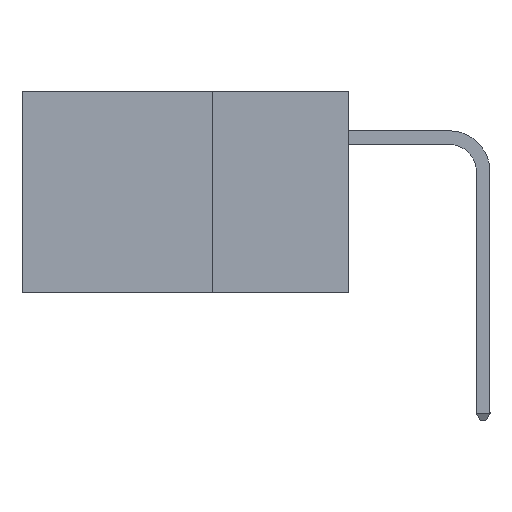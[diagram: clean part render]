
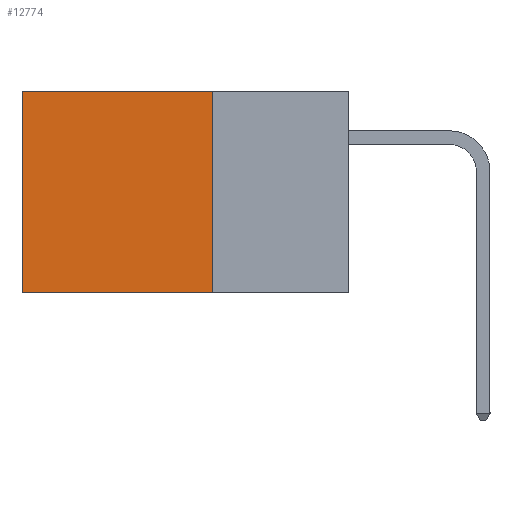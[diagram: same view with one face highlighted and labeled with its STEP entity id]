
A CAD part, left-side view. The second image highlights one B-rep face of the part: STEP entity #12774.
In plain terms, the highlighted planar face has unit normal (-1, 0, 0).
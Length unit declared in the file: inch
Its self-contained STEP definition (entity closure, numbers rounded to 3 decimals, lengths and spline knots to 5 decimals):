
#1997 = ORIENTED_EDGE ( 'NONE', *, *, #27370, .F. ) ;
#2489 = LINE ( 'NONE', #37557, #10954 ) ;
#5435 = CARTESIAN_POINT ( 'NONE',  ( 0.2875, 0.6, 0. ) ) ;
#5559 = VECTOR ( 'NONE', #21920, 39.37008 ) ;
#6791 = LINE ( 'NONE', #9286, #37528 ) ;
#7188 = AXIS2_PLACEMENT_3D ( 'NONE', #17265, #32128, #8507 ) ;
#7825 = EDGE_CURVE ( 'NONE', #21412, #36766, #33072, .T. ) ;
#8507 = DIRECTION ( 'NONE',  ( 0., 0., -1. ) ) ;
#9286 = CARTESIAN_POINT ( 'NONE',  ( 0.2875, 0.25, 0. ) ) ;
#10276 = CARTESIAN_POINT ( 'NONE',  ( 0.2875, 0.6, 0. ) ) ;
#10954 = VECTOR ( 'NONE', #14282, 39.37008 ) ;
#12774 = ADVANCED_FACE ( 'NONE', ( #19573 ), #25663, .F. ) ;
#14282 = DIRECTION ( 'NONE',  ( 0., 1., 0. ) ) ;
#15362 = EDGE_CURVE ( 'NONE', #36766, #19641, #24756, .T. ) ;
#17265 = CARTESIAN_POINT ( 'NONE',  ( 0.2875, 0.25, 0. ) ) ;
#18591 = DIRECTION ( 'NONE',  ( 0., 0., -1. ) ) ;
#19573 = FACE_OUTER_BOUND ( 'NONE', #32925, .T. ) ;
#19641 = VERTEX_POINT ( 'NONE', #34172 ) ;
#21412 = VERTEX_POINT ( 'NONE', #26914 ) ;
#21839 = CARTESIAN_POINT ( 'NONE',  ( 0.2875, 0.25, 0. ) ) ;
#21920 = DIRECTION ( 'NONE',  ( 0., 0., -1. ) ) ;
#23486 = EDGE_CURVE ( 'NONE', #21412, #24612, #6791, .T. ) ;
#24084 = ORIENTED_EDGE ( 'NONE', *, *, #23486, .F. ) ;
#24612 = VERTEX_POINT ( 'NONE', #30520 ) ;
#24756 = LINE ( 'NONE', #10276, #5559 ) ;
#25663 = PLANE ( 'NONE',  #7188 ) ;
#26505 = ORIENTED_EDGE ( 'NONE', *, *, #7825, .T. ) ;
#26914 = CARTESIAN_POINT ( 'NONE',  ( 0.2875, 0.25, 0. ) ) ;
#27370 = EDGE_CURVE ( 'NONE', #24612, #19641, #2489, .T. ) ;
#30520 = CARTESIAN_POINT ( 'NONE',  ( 0.2875, 0.25, -0.37 ) ) ;
#32128 = DIRECTION ( 'NONE',  ( 1., 0., 0. ) ) ;
#32925 = EDGE_LOOP ( 'NONE', ( #34605, #1997, #24084, #26505 ) ) ;
#33072 = LINE ( 'NONE', #21839, #36279 ) ;
#33633 = DIRECTION ( 'NONE',  ( 0., 1., 0. ) ) ;
#34172 = CARTESIAN_POINT ( 'NONE',  ( 0.2875, 0.6, -0.37 ) ) ;
#34605 = ORIENTED_EDGE ( 'NONE', *, *, #15362, .T. ) ;
#36279 = VECTOR ( 'NONE', #33633, 39.37008 ) ;
#36766 = VERTEX_POINT ( 'NONE', #5435 ) ;
#37528 = VECTOR ( 'NONE', #18591, 39.37008 ) ;
#37557 = CARTESIAN_POINT ( 'NONE',  ( 0.2875, 0.25, -0.37 ) ) ;
